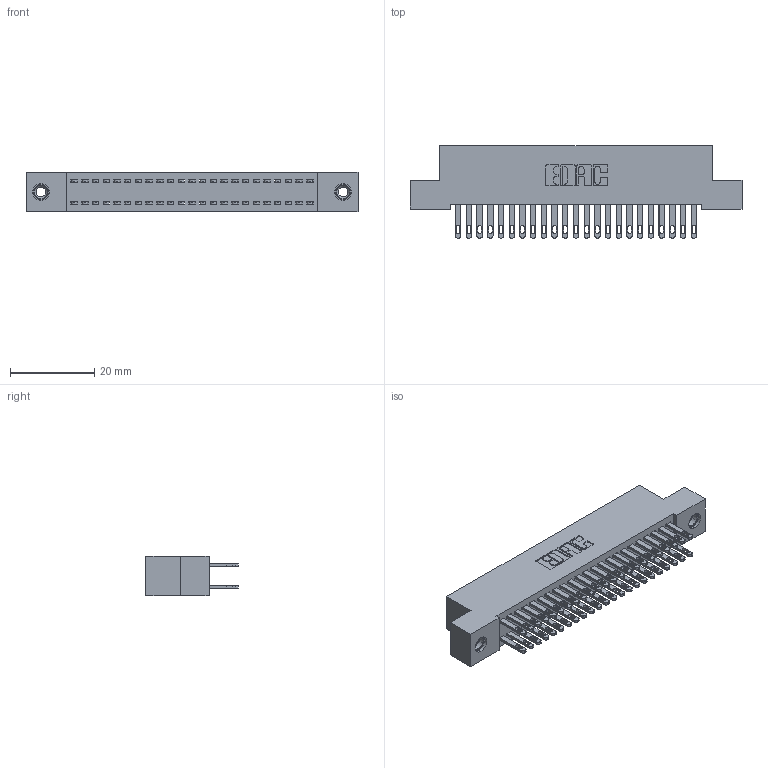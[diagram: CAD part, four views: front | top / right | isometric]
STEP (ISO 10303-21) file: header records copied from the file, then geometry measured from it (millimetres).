
FILE_DESCRIPTION (( 'STEP AP203' ), '1' );
FILE_NAME ('892-046-500-208.STEP', '2020-09-21T17:19:59', ( '' ), ( '' ), 'SwSTEP 2.0', 'SolidWorks 2020', '' );
FILE_SCHEMA (( 'CONFIG_CONTROL_DESIGN' ));
Length unit declared in the file: inch
Products named in the file (4): 842 Part_TI; 892-046-500-208; 345-250-001_345-250-003-102; 345-292-001_345-293-100
Assembly tree (49 placements, depth 2):
  892-046-500-208
    842 Part_TI
    345-292-001_345-293-100  x46
    345-250-001_345-250-003-102  x2
Bounding box: 78.74 x 21.85 x 9.4 mm (x, y, z)
Volume: 7119.7 mm3; surface area: 11571.7 mm2
Topology: 49 solids, 49 shells, 2378 faces, 7197 edges, 4790 vertices
Faces by surface type: plane 1478, cylinder 884, cone 12, torus 4
Entity records: 18238 total; most frequent: CARTESIAN_POINT 3025, ORIENTED_EDGE 2954, DIRECTION 2651, EDGE_CURVE 1477, VECTOR 1325, LINE 1325, VERTEX_POINT 980, AXIS2_PLACEMENT_3D 663
